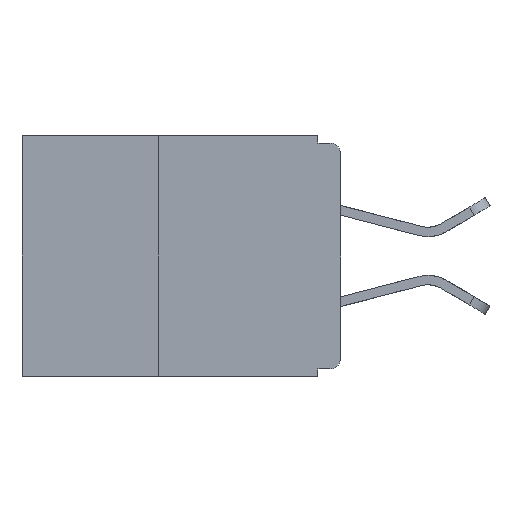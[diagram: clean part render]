
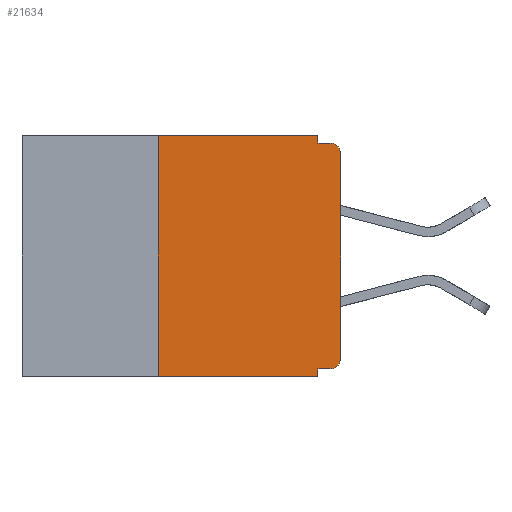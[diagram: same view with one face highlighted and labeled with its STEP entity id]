
A CAD part, left-side view. The second image highlights one B-rep face of the part: STEP entity #21634.
In plain terms, the highlighted planar face has unit normal (-1, 0, 0).
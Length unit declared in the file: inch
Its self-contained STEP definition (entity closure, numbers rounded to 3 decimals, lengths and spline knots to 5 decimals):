
#1048 = VECTOR ( 'NONE', #19393, 39.37008 ) ;
#1539 = VECTOR ( 'NONE', #4248, 39.37008 ) ;
#1660 = CARTESIAN_POINT ( 'NONE',  ( 0., 0.031, -0.33 ) ) ;
#1829 = VERTEX_POINT ( 'NONE', #19633 ) ;
#2343 = EDGE_CURVE ( 'NONE', #7597, #22983, #12491, .T. ) ;
#2466 = CARTESIAN_POINT ( 'NONE',  ( 0., 0.015, -0.025 ) ) ;
#2643 = CARTESIAN_POINT ( 'NONE',  ( 0., 0.25, -0.33 ) ) ;
#2670 = ORIENTED_EDGE ( 'NONE', *, *, #18072, .T. ) ;
#2851 = VECTOR ( 'NONE', #18735, 39.37008 ) ;
#3256 = EDGE_CURVE ( 'NONE', #1829, #8988, #22781, .T. ) ;
#3358 = DIRECTION ( 'NONE',  ( 0., 1., 0. ) ) ;
#3374 = LINE ( 'NONE', #22405, #23218 ) ;
#3689 = CARTESIAN_POINT ( 'NONE',  ( 0., 0.015, -0.305 ) ) ;
#3824 = EDGE_CURVE ( 'NONE', #7597, #8988, #6086, .T. ) ;
#4172 = CARTESIAN_POINT ( 'NONE',  ( 0., 0.437, 0. ) ) ;
#4248 = DIRECTION ( 'NONE',  ( 0., -1., 0. ) ) ;
#4368 = DIRECTION ( 'NONE',  ( 0., 0., -1. ) ) ;
#4987 = CARTESIAN_POINT ( 'NONE',  ( 0., 0., -0.305 ) ) ;
#5248 = CARTESIAN_POINT ( 'NONE',  ( 0., 0.031, 0. ) ) ;
#5488 = EDGE_CURVE ( 'NONE', #23646, #13773, #3374, .T. ) ;
#5536 = DIRECTION ( 'NONE',  ( 0., 0., -1. ) ) ;
#5949 = CARTESIAN_POINT ( 'NONE',  ( 0., 0., 0. ) ) ;
#5998 = EDGE_CURVE ( 'NONE', #22983, #10182, #7133, .T. ) ;
#6086 = LINE ( 'NONE', #20319, #1048 ) ;
#6661 = VERTEX_POINT ( 'NONE', #21879 ) ;
#6668 = ORIENTED_EDGE ( 'NONE', *, *, #2343, .F. ) ;
#6982 = CARTESIAN_POINT ( 'NONE',  ( 0., 0.437, 0. ) ) ;
#7133 = LINE ( 'NONE', #4172, #1539 ) ;
#7531 = VERTEX_POINT ( 'NONE', #4987 ) ;
#7597 = VERTEX_POINT ( 'NONE', #2643 ) ;
#7803 = CIRCLE ( 'NONE', #8981, 0.015 ) ;
#8775 = CARTESIAN_POINT ( 'NONE',  ( 0., 0.015, -0.01 ) ) ;
#8807 = DIRECTION ( 'NONE',  ( 0., 0., -1. ) ) ;
#8981 = AXIS2_PLACEMENT_3D ( 'NONE', #2466, #15390, #4368 ) ;
#8988 = VERTEX_POINT ( 'NONE', #11971 ) ;
#9314 = CARTESIAN_POINT ( 'NONE',  ( 0., 0., -0.025 ) ) ;
#9804 = ORIENTED_EDGE ( 'NONE', *, *, #3824, .T. ) ;
#10182 = VERTEX_POINT ( 'NONE', #11603 ) ;
#11417 = AXIS2_PLACEMENT_3D ( 'NONE', #6982, #19658, #8807 ) ;
#11603 = CARTESIAN_POINT ( 'NONE',  ( 0., 0.031, 0. ) ) ;
#11971 = CARTESIAN_POINT ( 'NONE',  ( 0., 0.031, -0.33 ) ) ;
#11988 = CARTESIAN_POINT ( 'NONE',  ( 0., 0.031, -0.01 ) ) ;
#12053 = ORIENTED_EDGE ( 'NONE', *, *, #16469, .T. ) ;
#12357 = ORIENTED_EDGE ( 'NONE', *, *, #17136, .T. ) ;
#12491 = LINE ( 'NONE', #17638, #17276 ) ;
#12766 = VECTOR ( 'NONE', #3358, 39.37008 ) ;
#12925 = FACE_OUTER_BOUND ( 'NONE', #13931, .T. ) ;
#13382 = CARTESIAN_POINT ( 'NONE',  ( 0., 0.25, 0. ) ) ;
#13773 = VERTEX_POINT ( 'NONE', #8775 ) ;
#13931 = EDGE_LOOP ( 'NONE', ( #12053, #12357, #14360, #18382, #21929, #6668, #9804, #20253, #22792, #2670 ) ) ;
#13984 = LINE ( 'NONE', #5248, #18193 ) ;
#14360 = ORIENTED_EDGE ( 'NONE', *, *, #5488, .F. ) ;
#14517 = DIRECTION ( 'NONE',  ( 0., 0., 1. ) ) ;
#15390 = DIRECTION ( 'NONE',  ( -1., 0., 0. ) ) ;
#15598 = EDGE_CURVE ( 'NONE', #6661, #1829, #22780, .T. ) ;
#16230 = CARTESIAN_POINT ( 'NONE',  ( 0., 0., -0.32 ) ) ;
#16325 = DIRECTION ( 'NONE',  ( 0., 0., -1. ) ) ;
#16469 = EDGE_CURVE ( 'NONE', #7531, #16981, #17512, .T. ) ;
#16546 = DIRECTION ( 'NONE',  ( -1., 0., 0. ) ) ;
#16981 = VERTEX_POINT ( 'NONE', #9314 ) ;
#17136 = EDGE_CURVE ( 'NONE', #16981, #13773, #7803, .T. ) ;
#17276 = VECTOR ( 'NONE', #14517, 39.37008 ) ;
#17512 = LINE ( 'NONE', #5949, #2851 ) ;
#17638 = CARTESIAN_POINT ( 'NONE',  ( 0., 0.25, -0.33 ) ) ;
#17911 = PLANE ( 'NONE',  #11417 ) ;
#18072 = EDGE_CURVE ( 'NONE', #6661, #7531, #21037, .T. ) ;
#18083 = DIRECTION ( 'NONE',  ( 0., 0., -1. ) ) ;
#18193 = VECTOR ( 'NONE', #18083, 39.37008 ) ;
#18382 = ORIENTED_EDGE ( 'NONE', *, *, #23345, .F. ) ;
#18613 = AXIS2_PLACEMENT_3D ( 'NONE', #3689, #16546, #5536 ) ;
#18735 = DIRECTION ( 'NONE',  ( 0., 0., 1. ) ) ;
#19393 = DIRECTION ( 'NONE',  ( 0., -1., 0. ) ) ;
#19633 = CARTESIAN_POINT ( 'NONE',  ( 0., 0.031, -0.32 ) ) ;
#19658 = DIRECTION ( 'NONE',  ( 1., 0., 0. ) ) ;
#20253 = ORIENTED_EDGE ( 'NONE', *, *, #3256, .F. ) ;
#20319 = CARTESIAN_POINT ( 'NONE',  ( 0., 0.437, -0.33 ) ) ;
#21037 = CIRCLE ( 'NONE', #18613, 0.015 ) ;
#21634 = ADVANCED_FACE ( 'NONE', ( #12925 ), #17911, .F. ) ;
#21879 = CARTESIAN_POINT ( 'NONE',  ( 0., 0.015, -0.32 ) ) ;
#21929 = ORIENTED_EDGE ( 'NONE', *, *, #5998, .F. ) ;
#22329 = DIRECTION ( 'NONE',  ( 0., -1., 0. ) ) ;
#22405 = CARTESIAN_POINT ( 'NONE',  ( 0., 0., -0.01 ) ) ;
#22780 = LINE ( 'NONE', #16230, #12766 ) ;
#22781 = LINE ( 'NONE', #1660, #23336 ) ;
#22792 = ORIENTED_EDGE ( 'NONE', *, *, #15598, .F. ) ;
#22983 = VERTEX_POINT ( 'NONE', #13382 ) ;
#23218 = VECTOR ( 'NONE', #22329, 39.37008 ) ;
#23336 = VECTOR ( 'NONE', #16325, 39.37008 ) ;
#23345 = EDGE_CURVE ( 'NONE', #10182, #23646, #13984, .T. ) ;
#23646 = VERTEX_POINT ( 'NONE', #11988 ) ;
